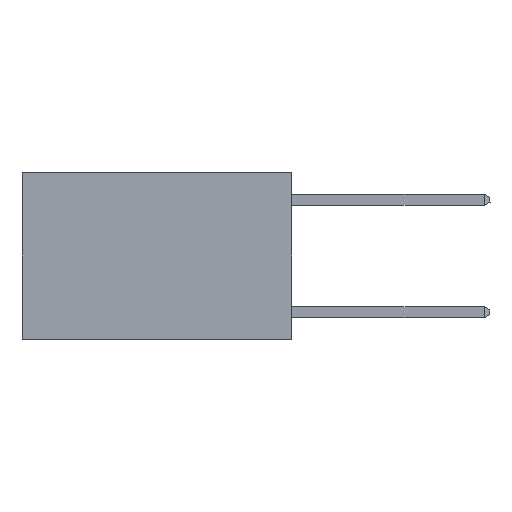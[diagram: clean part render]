
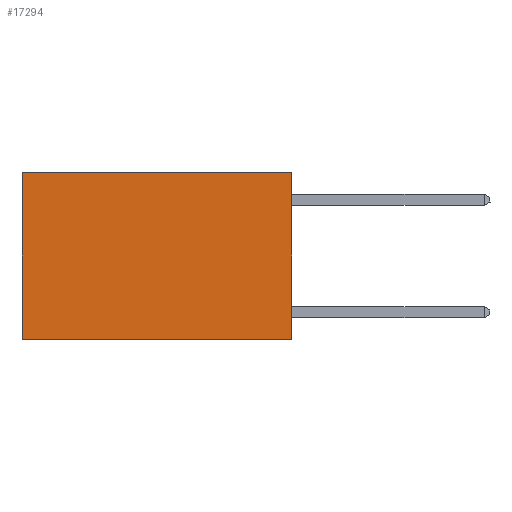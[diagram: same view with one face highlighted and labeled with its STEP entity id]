
A CAD part, left-side view. The second image highlights one B-rep face of the part: STEP entity #17294.
In plain terms, the highlighted planar face has unit normal (-1, 0, 0).
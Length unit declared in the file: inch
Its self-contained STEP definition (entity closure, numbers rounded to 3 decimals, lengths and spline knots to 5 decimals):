
#1480 = VERTEX_POINT ( 'NONE', #5366 ) ;
#1652 = CARTESIAN_POINT ( 'NONE',  ( 0.2625, 0., -0.37 ) ) ;
#2580 = DIRECTION ( 'NONE',  ( 0., 0., -1. ) ) ;
#3039 = DIRECTION ( 'NONE',  ( 0., 0., -1. ) ) ;
#3537 = EDGE_LOOP ( 'NONE', ( #15915, #16064, #14287, #17888 ) ) ;
#3995 = LINE ( 'NONE', #6018, #13624 ) ;
#5366 = CARTESIAN_POINT ( 'NONE',  ( 0.2625, 0.6, -0.37 ) ) ;
#5766 = VERTEX_POINT ( 'NONE', #1652 ) ;
#6018 = CARTESIAN_POINT ( 'NONE',  ( 0.2625, 0.6, 0. ) ) ;
#7138 = LINE ( 'NONE', #11890, #19118 ) ;
#7202 = EDGE_CURVE ( 'NONE', #12674, #1480, #3995, .T. ) ;
#7952 = LINE ( 'NONE', #13212, #17544 ) ;
#8512 = DIRECTION ( 'NONE',  ( 0., 1., 0. ) ) ;
#8610 = FACE_OUTER_BOUND ( 'NONE', #3537, .T. ) ;
#9366 = CARTESIAN_POINT ( 'NONE',  ( 0.2625, 0.6, 0. ) ) ;
#9427 = EDGE_CURVE ( 'NONE', #9729, #12674, #7952, .T. ) ;
#9729 = VERTEX_POINT ( 'NONE', #15822 ) ;
#10218 = DIRECTION ( 'NONE',  ( 1., 0., 0. ) ) ;
#11284 = CARTESIAN_POINT ( 'NONE',  ( 0.2625, 0., -0.37 ) ) ;
#11890 = CARTESIAN_POINT ( 'NONE',  ( 0.2625, 0., 0. ) ) ;
#12674 = VERTEX_POINT ( 'NONE', #9366 ) ;
#13212 = CARTESIAN_POINT ( 'NONE',  ( 0.2625, 0., 0. ) ) ;
#13624 = VECTOR ( 'NONE', #3039, 39.37008 ) ;
#14122 = EDGE_CURVE ( 'NONE', #9729, #5766, #7138, .T. ) ;
#14287 = ORIENTED_EDGE ( 'NONE', *, *, #14122, .F. ) ;
#14478 = EDGE_CURVE ( 'NONE', #5766, #1480, #18310, .T. ) ;
#14688 = PLANE ( 'NONE',  #15896 ) ;
#15822 = CARTESIAN_POINT ( 'NONE',  ( 0.2625, 0., 0. ) ) ;
#15896 = AXIS2_PLACEMENT_3D ( 'NONE', #19423, #10218, #2580 ) ;
#15915 = ORIENTED_EDGE ( 'NONE', *, *, #7202, .T. ) ;
#16064 = ORIENTED_EDGE ( 'NONE', *, *, #14478, .F. ) ;
#16655 = VECTOR ( 'NONE', #17471, 39.37008 ) ;
#17294 = ADVANCED_FACE ( 'NONE', ( #8610 ), #14688, .F. ) ;
#17471 = DIRECTION ( 'NONE',  ( 0., 1., 0. ) ) ;
#17544 = VECTOR ( 'NONE', #8512, 39.37008 ) ;
#17888 = ORIENTED_EDGE ( 'NONE', *, *, #9427, .T. ) ;
#18310 = LINE ( 'NONE', #11284, #16655 ) ;
#19118 = VECTOR ( 'NONE', #19675, 39.37008 ) ;
#19423 = CARTESIAN_POINT ( 'NONE',  ( 0.2625, 0., 0. ) ) ;
#19675 = DIRECTION ( 'NONE',  ( 0., 0., -1. ) ) ;
